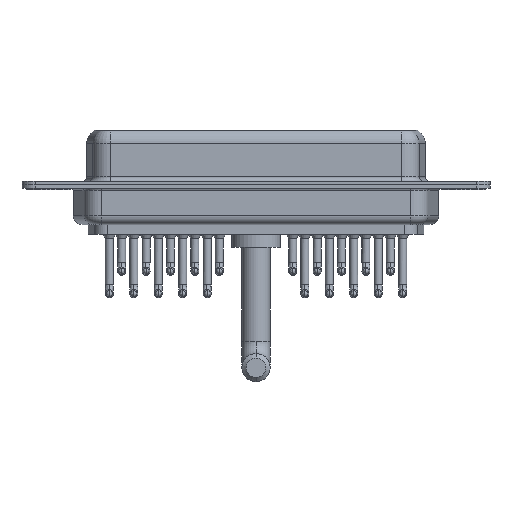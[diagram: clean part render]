
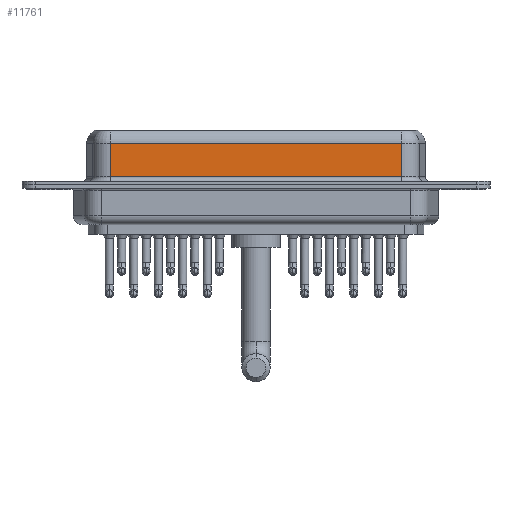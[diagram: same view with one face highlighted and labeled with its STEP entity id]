
A CAD part, front view. The second image highlights one B-rep face of the part: STEP entity #11761.
In plain terms, the highlighted planar face has unit normal (0, -1, 0).
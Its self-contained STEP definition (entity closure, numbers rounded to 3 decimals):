
#1418 = DIRECTION ( 'NONE',  ( 0., 0., 1. ) ) ;
#1793 = LINE ( 'NONE', #19643, #7760 ) ;
#3474 = DIRECTION ( 'NONE',  ( -1., 0., 0. ) ) ;
#3595 = DIRECTION ( 'NONE',  ( 0., 0., -1. ) ) ;
#4588 = ORIENTED_EDGE ( 'NONE', *, *, #8836, .T. ) ;
#4681 = CARTESIAN_POINT ( 'NONE',  ( 40.037, -3.95, 6.4 ) ) ;
#5342 = ORIENTED_EDGE ( 'NONE', *, *, #9783, .T. ) ;
#5792 = LINE ( 'NONE', #6199, #8714 ) ;
#6018 = VECTOR ( 'NONE', #19424, 1000. ) ;
#6199 = CARTESIAN_POINT ( 'NONE',  ( 40.037, -3.95, 0.9 ) ) ;
#7194 = VERTEX_POINT ( 'NONE', #11105 ) ;
#7760 = VECTOR ( 'NONE', #3474, 1000. ) ;
#8047 = LINE ( 'NONE', #9931, #20238 ) ;
#8714 = VECTOR ( 'NONE', #18912, 1000. ) ;
#8836 = EDGE_CURVE ( 'NONE', #9340, #13101, #18053, .T. ) ;
#8918 = VERTEX_POINT ( 'NONE', #20051 ) ;
#9340 = VERTEX_POINT ( 'NONE', #20030 ) ;
#9458 = PLANE ( 'NONE',  #10021 ) ;
#9783 = EDGE_CURVE ( 'NONE', #13101, #7194, #5792, .T. ) ;
#9931 = CARTESIAN_POINT ( 'NONE',  ( 40.037, -3.95, 6.4 ) ) ;
#10021 = AXIS2_PLACEMENT_3D ( 'NONE', #4681, #15900, #1418 ) ;
#11105 = CARTESIAN_POINT ( 'NONE',  ( 40.037, -3.95, 0.9 ) ) ;
#11761 = ADVANCED_FACE ( 'NONE', ( #17475 ), #9458, .F. ) ;
#13101 = VERTEX_POINT ( 'NONE', #18098 ) ;
#14566 = CARTESIAN_POINT ( 'NONE',  ( 7.013, -3.95, 6.4 ) ) ;
#14889 = EDGE_CURVE ( 'NONE', #8918, #9340, #1793, .T. ) ;
#15900 = DIRECTION ( 'NONE',  ( 0., 1., 0. ) ) ;
#16978 = ORIENTED_EDGE ( 'NONE', *, *, #14889, .T. ) ;
#17475 = FACE_OUTER_BOUND ( 'NONE', #19158, .T. ) ;
#18053 = LINE ( 'NONE', #14566, #6018 ) ;
#18098 = CARTESIAN_POINT ( 'NONE',  ( 7.013, -3.95, 0.9 ) ) ;
#18579 = ORIENTED_EDGE ( 'NONE', *, *, #19972, .F. ) ;
#18912 = DIRECTION ( 'NONE',  ( 1., 0., 0. ) ) ;
#19158 = EDGE_LOOP ( 'NONE', ( #18579, #16978, #4588, #5342 ) ) ;
#19424 = DIRECTION ( 'NONE',  ( 0., 0., -1. ) ) ;
#19643 = CARTESIAN_POINT ( 'NONE',  ( 40.037, -3.95, 4.65 ) ) ;
#19972 = EDGE_CURVE ( 'NONE', #8918, #7194, #8047, .T. ) ;
#20030 = CARTESIAN_POINT ( 'NONE',  ( 7.013, -3.95, 4.65 ) ) ;
#20051 = CARTESIAN_POINT ( 'NONE',  ( 40.037, -3.95, 4.65 ) ) ;
#20238 = VECTOR ( 'NONE', #3595, 1000. ) ;
